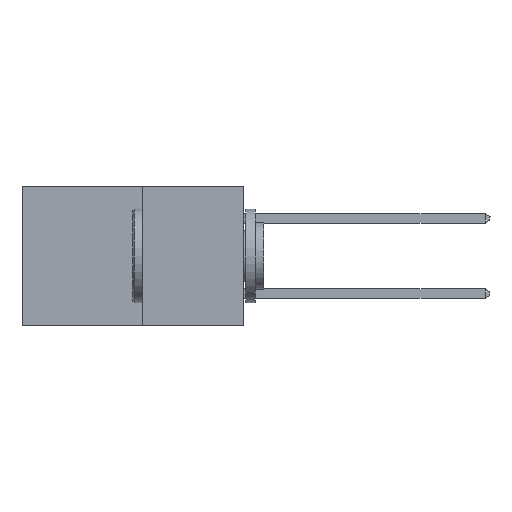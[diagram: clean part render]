
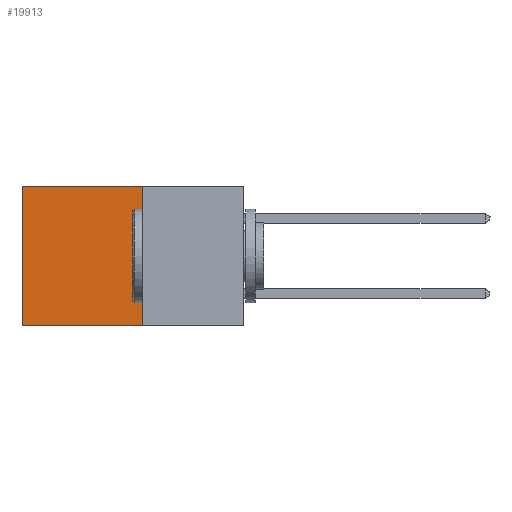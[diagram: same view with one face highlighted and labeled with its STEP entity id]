
A CAD part, left-side view. The second image highlights one B-rep face of the part: STEP entity #19913.
In plain terms, the highlighted planar face has unit normal (-1, 0, 0).
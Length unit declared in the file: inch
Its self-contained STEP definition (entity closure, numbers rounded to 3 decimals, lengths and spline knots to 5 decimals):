
#1393 = ORIENTED_EDGE ( 'NONE', *, *, #19592, .T. ) ;
#2033 = DIRECTION ( 'NONE',  ( 0., 0., -1. ) ) ;
#2596 = LINE ( 'NONE', #17279, #10085 ) ;
#2874 = FACE_OUTER_BOUND ( 'NONE', #5388, .T. ) ;
#2955 = CARTESIAN_POINT ( 'NONE',  ( 0.277, 0.59, 0. ) ) ;
#3850 = AXIS2_PLACEMENT_3D ( 'NONE', #8374, #11549, #2033 ) ;
#5151 = ORIENTED_EDGE ( 'NONE', *, *, #13688, .F. ) ;
#5388 = EDGE_LOOP ( 'NONE', ( #17225, #5151, #9375, #1393 ) ) ;
#5567 = CARTESIAN_POINT ( 'NONE',  ( 0.277, 0.59, -0.37 ) ) ;
#6038 = EDGE_CURVE ( 'NONE', #18737, #16928, #20199, .T. ) ;
#6064 = CARTESIAN_POINT ( 'NONE',  ( 0.277, 0.27, 0. ) ) ;
#6842 = PLANE ( 'NONE',  #3850 ) ;
#6977 = CARTESIAN_POINT ( 'NONE',  ( 0.277, 0.27, -0.37 ) ) ;
#7921 = DIRECTION ( 'NONE',  ( 0., 0., -1. ) ) ;
#8374 = CARTESIAN_POINT ( 'NONE',  ( 0.277, 0.27, -0.37 ) ) ;
#8548 = DIRECTION ( 'NONE',  ( 0., 1., 0. ) ) ;
#9107 = VERTEX_POINT ( 'NONE', #2955 ) ;
#9375 = ORIENTED_EDGE ( 'NONE', *, *, #6038, .F. ) ;
#9862 = VECTOR ( 'NONE', #17028, 39.37008 ) ;
#10085 = VECTOR ( 'NONE', #7921, 39.37008 ) ;
#10374 = CARTESIAN_POINT ( 'NONE',  ( 0.277, 0.27, 0. ) ) ;
#11549 = DIRECTION ( 'NONE',  ( 1., 0., 0. ) ) ;
#13173 = VERTEX_POINT ( 'NONE', #5567 ) ;
#13311 = VECTOR ( 'NONE', #8548, 39.37008 ) ;
#13688 = EDGE_CURVE ( 'NONE', #16928, #13173, #18029, .T. ) ;
#13978 = LINE ( 'NONE', #6064, #9862 ) ;
#14792 = CARTESIAN_POINT ( 'NONE',  ( 0.277, 0.27, -0.37 ) ) ;
#16928 = VERTEX_POINT ( 'NONE', #14792 ) ;
#16937 = DIRECTION ( 'NONE',  ( 0., 0., -1. ) ) ;
#16980 = CARTESIAN_POINT ( 'NONE',  ( 0.277, 0.27, -0.37 ) ) ;
#17028 = DIRECTION ( 'NONE',  ( 0., 1., 0. ) ) ;
#17225 = ORIENTED_EDGE ( 'NONE', *, *, #20180, .T. ) ;
#17279 = CARTESIAN_POINT ( 'NONE',  ( 0.277, 0.59, -0.37 ) ) ;
#18029 = LINE ( 'NONE', #6977, #13311 ) ;
#18737 = VERTEX_POINT ( 'NONE', #10374 ) ;
#19592 = EDGE_CURVE ( 'NONE', #18737, #9107, #13978, .T. ) ;
#19743 = VECTOR ( 'NONE', #16937, 39.37008 ) ;
#19913 = ADVANCED_FACE ( 'NONE', ( #2874 ), #6842, .F. ) ;
#20180 = EDGE_CURVE ( 'NONE', #9107, #13173, #2596, .T. ) ;
#20199 = LINE ( 'NONE', #16980, #19743 ) ;
